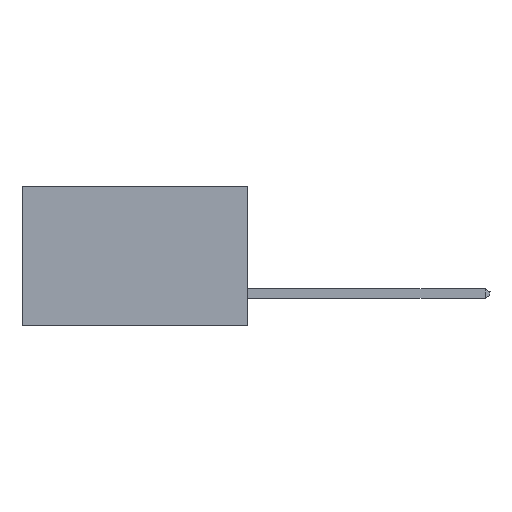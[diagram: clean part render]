
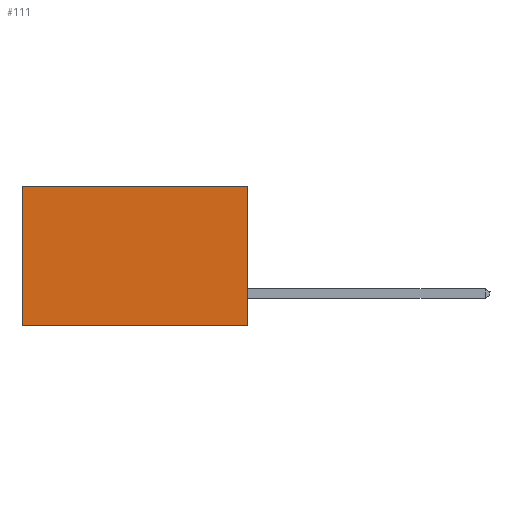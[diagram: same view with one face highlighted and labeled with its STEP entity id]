
A CAD part, left-side view. The second image highlights one B-rep face of the part: STEP entity #111.
In plain terms, the highlighted planar face has unit normal (-1, 0, 0).
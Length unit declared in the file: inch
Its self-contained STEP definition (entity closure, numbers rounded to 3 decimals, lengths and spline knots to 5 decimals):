
#93 = CARTESIAN_POINT ( 'NONE',  ( 0.2615, 0.6, -0.37 ) ) ;
#111 = ADVANCED_FACE ( 'NONE', ( #9520 ), #11995, .F. ) ;
#862 = DIRECTION ( 'NONE',  ( 1., 0., 0. ) ) ;
#1527 = CARTESIAN_POINT ( 'NONE',  ( 0.2615, 0., 0. ) ) ;
#1605 = VECTOR ( 'NONE', #18904, 39.37008 ) ;
#2516 = VERTEX_POINT ( 'NONE', #4025 ) ;
#2984 = CARTESIAN_POINT ( 'NONE',  ( 0.2615, 0., -0.37 ) ) ;
#4025 = CARTESIAN_POINT ( 'NONE',  ( 0.2615, 0., -0.37 ) ) ;
#5452 = EDGE_CURVE ( 'NONE', #18402, #21941, #14414, .T. ) ;
#5876 = VECTOR ( 'NONE', #13772, 39.37008 ) ;
#6857 = EDGE_CURVE ( 'NONE', #2516, #13513, #7328, .T. ) ;
#6990 = DIRECTION ( 'NONE',  ( 0., 1., 0. ) ) ;
#7328 = LINE ( 'NONE', #13838, #12688 ) ;
#7539 = ORIENTED_EDGE ( 'NONE', *, *, #10596, .F. ) ;
#8788 = EDGE_CURVE ( 'NONE', #21941, #13513, #15490, .T. ) ;
#9520 = FACE_OUTER_BOUND ( 'NONE', #21874, .T. ) ;
#10173 = DIRECTION ( 'NONE',  ( 0., 0., -1. ) ) ;
#10596 = EDGE_CURVE ( 'NONE', #18402, #2516, #11929, .T. ) ;
#11084 = AXIS2_PLACEMENT_3D ( 'NONE', #2984, #862, #10173 ) ;
#11906 = CARTESIAN_POINT ( 'NONE',  ( 0.2615, 0.6, -0.37 ) ) ;
#11929 = LINE ( 'NONE', #15691, #1605 ) ;
#11995 = PLANE ( 'NONE',  #11084 ) ;
#12688 = VECTOR ( 'NONE', #6990, 39.37008 ) ;
#13513 = VERTEX_POINT ( 'NONE', #11906 ) ;
#13772 = DIRECTION ( 'NONE',  ( 0., 0., -1. ) ) ;
#13838 = CARTESIAN_POINT ( 'NONE',  ( 0.2615, 0., -0.37 ) ) ;
#14414 = LINE ( 'NONE', #1527, #21848 ) ;
#14804 = ORIENTED_EDGE ( 'NONE', *, *, #8788, .T. ) ;
#15209 = DIRECTION ( 'NONE',  ( 0., 1., 0. ) ) ;
#15490 = LINE ( 'NONE', #93, #5876 ) ;
#15691 = CARTESIAN_POINT ( 'NONE',  ( 0.2615, 0., -0.37 ) ) ;
#16453 = CARTESIAN_POINT ( 'NONE',  ( 0.2615, 0.6, 0. ) ) ;
#17100 = ORIENTED_EDGE ( 'NONE', *, *, #6857, .F. ) ;
#18402 = VERTEX_POINT ( 'NONE', #22291 ) ;
#18904 = DIRECTION ( 'NONE',  ( 0., 0., -1. ) ) ;
#20766 = ORIENTED_EDGE ( 'NONE', *, *, #5452, .T. ) ;
#21848 = VECTOR ( 'NONE', #15209, 39.37008 ) ;
#21874 = EDGE_LOOP ( 'NONE', ( #14804, #17100, #7539, #20766 ) ) ;
#21941 = VERTEX_POINT ( 'NONE', #16453 ) ;
#22291 = CARTESIAN_POINT ( 'NONE',  ( 0.2615, 0., 0. ) ) ;
